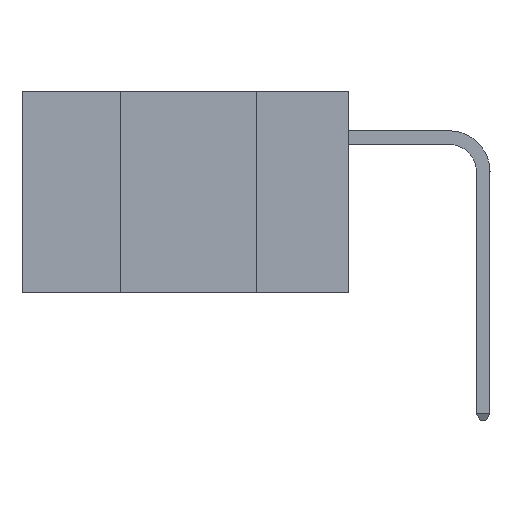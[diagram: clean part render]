
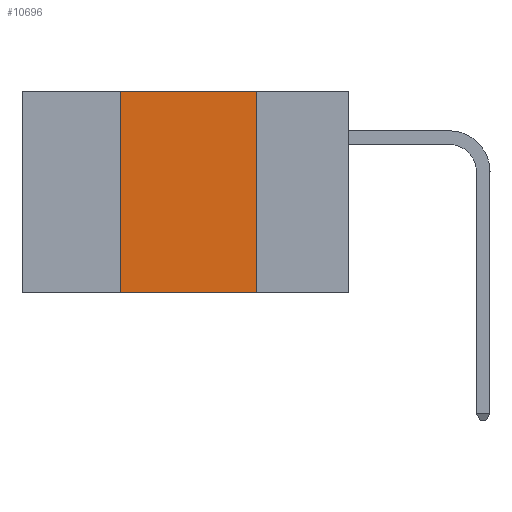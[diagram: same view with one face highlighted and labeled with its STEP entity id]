
A CAD part, left-side view. The second image highlights one B-rep face of the part: STEP entity #10696.
In plain terms, the highlighted planar face has unit normal (-1, 0, 0).
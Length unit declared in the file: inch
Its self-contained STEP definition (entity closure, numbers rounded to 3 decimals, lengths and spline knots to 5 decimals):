
#69 = EDGE_CURVE ( 'NONE', #16630, #14746, #12895, .T. ) ;
#1802 = CARTESIAN_POINT ( 'NONE',  ( 0., 0.6, -0.37 ) ) ;
#2154 = ORIENTED_EDGE ( 'NONE', *, *, #3585, .F. ) ;
#3271 = EDGE_CURVE ( 'NONE', #14746, #14711, #6482, .T. ) ;
#3386 = AXIS2_PLACEMENT_3D ( 'NONE', #5438, #6991, #17256 ) ;
#3413 = DIRECTION ( 'NONE',  ( 0., -1., 0. ) ) ;
#3459 = CARTESIAN_POINT ( 'NONE',  ( 0., 0.17, 0. ) ) ;
#3585 = EDGE_CURVE ( 'NONE', #14711, #6416, #17498, .T. ) ;
#4015 = EDGE_LOOP ( 'NONE', ( #2154, #18941, #12589, #6060 ) ) ;
#4187 = LINE ( 'NONE', #1802, #11678 ) ;
#4206 = FACE_OUTER_BOUND ( 'NONE', #4015, .T. ) ;
#5438 = CARTESIAN_POINT ( 'NONE',  ( 0., 0.6, 0. ) ) ;
#5742 = VECTOR ( 'NONE', #7335, 39.37008 ) ;
#6060 = ORIENTED_EDGE ( 'NONE', *, *, #11126, .T. ) ;
#6416 = VERTEX_POINT ( 'NONE', #15749 ) ;
#6482 = LINE ( 'NONE', #14033, #17744 ) ;
#6991 = DIRECTION ( 'NONE',  ( 1., 0., 0. ) ) ;
#7335 = DIRECTION ( 'NONE',  ( 0., 0., -1. ) ) ;
#8228 = DIRECTION ( 'NONE',  ( 0., -1., 0. ) ) ;
#9002 = VECTOR ( 'NONE', #17595, 39.37008 ) ;
#9428 = CARTESIAN_POINT ( 'NONE',  ( 0., 0.42, 0. ) ) ;
#9646 = CARTESIAN_POINT ( 'NONE',  ( 0., 0.42, 0. ) ) ;
#10696 = ADVANCED_FACE ( 'NONE', ( #4206 ), #14344, .F. ) ;
#11126 = EDGE_CURVE ( 'NONE', #16630, #6416, #4187, .T. ) ;
#11678 = VECTOR ( 'NONE', #3413, 39.37008 ) ;
#12589 = ORIENTED_EDGE ( 'NONE', *, *, #69, .F. ) ;
#12895 = LINE ( 'NONE', #9428, #9002 ) ;
#13205 = CARTESIAN_POINT ( 'NONE',  ( 0., 0.17, 0. ) ) ;
#14033 = CARTESIAN_POINT ( 'NONE',  ( 0., 0.6, 0. ) ) ;
#14344 = PLANE ( 'NONE',  #3386 ) ;
#14711 = VERTEX_POINT ( 'NONE', #3459 ) ;
#14746 = VERTEX_POINT ( 'NONE', #9646 ) ;
#15749 = CARTESIAN_POINT ( 'NONE',  ( 0., 0.17, -0.37 ) ) ;
#16630 = VERTEX_POINT ( 'NONE', #17998 ) ;
#17256 = DIRECTION ( 'NONE',  ( 0., 0., -1. ) ) ;
#17498 = LINE ( 'NONE', #13205, #5742 ) ;
#17595 = DIRECTION ( 'NONE',  ( 0., 0., 1. ) ) ;
#17744 = VECTOR ( 'NONE', #8228, 39.37008 ) ;
#17998 = CARTESIAN_POINT ( 'NONE',  ( 0., 0.42, -0.37 ) ) ;
#18941 = ORIENTED_EDGE ( 'NONE', *, *, #3271, .F. ) ;
